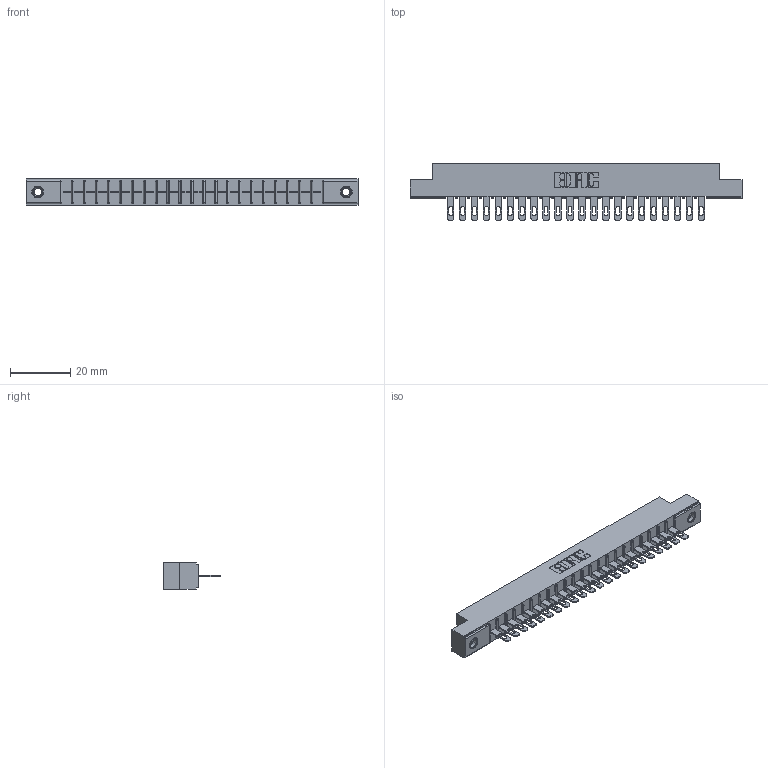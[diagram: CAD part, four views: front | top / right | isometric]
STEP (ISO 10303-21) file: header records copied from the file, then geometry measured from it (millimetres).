
FILE_DESCRIPTION (( 'STEP AP203' ), '1' );
FILE_NAME ('316-022-400-107.STEP', '2020-09-22T20:21:07', ( '' ), ( '' ), 'SwSTEP 2.0', 'SolidWorks 2020', '' );
FILE_SCHEMA (( 'CONFIG_CONTROL_DESIGN' ));
Length unit declared in the file: inch
Products named in the file (4): 345-250-001_345-250-005-103; 306-290-001_100; 316-022-400-107; 306 Part_.156 Dia
Assembly tree (25 placements, depth 2):
  316-022-400-107
    306 Part_.156 Dia
    306-290-001_100  x22
    345-250-001_345-250-005-103  x2
Bounding box: 110.19 x 18.87 x 8.71 mm (x, y, z)
Volume: 7597 mm3; surface area: 11612.2 mm2
Topology: 25 solids, 25 shells, 1848 faces, 5182 edges, 3328 vertices
Faces by surface type: plane 1200, cylinder 544, sphere 88, cone 12, torus 4
Entity records: 24456 total; most frequent: CARTESIAN_POINT 4084, ORIENTED_EDGE 4040, DIRECTION 4038, EDGE_CURVE 2020, VECTOR 1566, LINE 1566, VERTEX_POINT 1282, AXIS2_PLACEMENT_3D 1236
